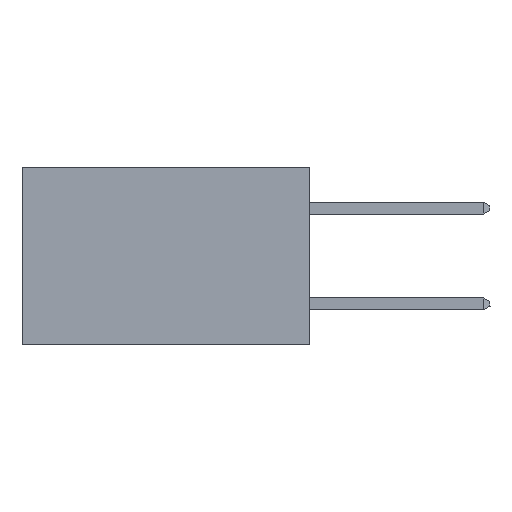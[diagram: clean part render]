
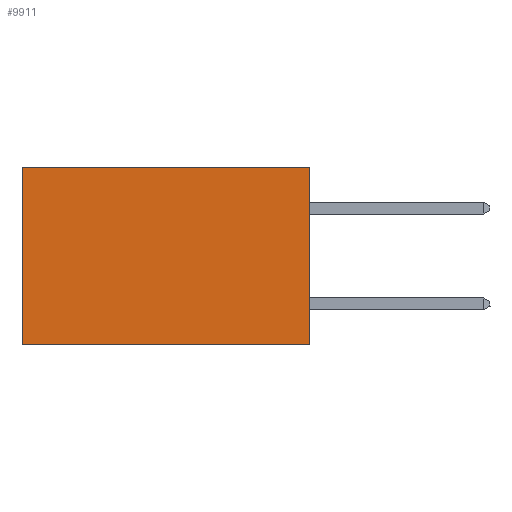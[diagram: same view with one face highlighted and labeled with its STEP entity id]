
A CAD part, left-side view. The second image highlights one B-rep face of the part: STEP entity #9911.
In plain terms, the highlighted planar face has unit normal (-1, 0, 0).
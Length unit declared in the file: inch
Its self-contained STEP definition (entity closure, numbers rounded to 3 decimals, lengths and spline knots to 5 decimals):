
#1926 = VECTOR ( 'NONE', #7332, 39.37008 ) ;
#2102 = EDGE_LOOP ( 'NONE', ( #9820, #22563, #12753, #5628 ) ) ;
#2512 = CARTESIAN_POINT ( 'NONE',  ( 0.2875, 0., 0. ) ) ;
#2703 = VERTEX_POINT ( 'NONE', #6665 ) ;
#3456 = LINE ( 'NONE', #10972, #8650 ) ;
#4264 = EDGE_CURVE ( 'NONE', #2703, #23102, #3456, .T. ) ;
#4873 = CARTESIAN_POINT ( 'NONE',  ( 0.2875, 0.6, -0.37 ) ) ;
#5211 = LINE ( 'NONE', #26821, #21614 ) ;
#5628 = ORIENTED_EDGE ( 'NONE', *, *, #11173, .T. ) ;
#6344 = VECTOR ( 'NONE', #9142, 39.37008 ) ;
#6665 = CARTESIAN_POINT ( 'NONE',  ( 0.2875, 0., -0.37 ) ) ;
#7332 = DIRECTION ( 'NONE',  ( 0., 0., -1. ) ) ;
#8149 = FACE_OUTER_BOUND ( 'NONE', #2102, .T. ) ;
#8650 = VECTOR ( 'NONE', #13106, 39.37008 ) ;
#9142 = DIRECTION ( 'NONE',  ( 0., 1., 0. ) ) ;
#9820 = ORIENTED_EDGE ( 'NONE', *, *, #18787, .T. ) ;
#9911 = ADVANCED_FACE ( 'NONE', ( #8149 ), #19847, .F. ) ;
#10972 = CARTESIAN_POINT ( 'NONE',  ( 0.2875, 0., -0.37 ) ) ;
#11173 = EDGE_CURVE ( 'NONE', #26231, #19776, #12278, .T. ) ;
#12278 = LINE ( 'NONE', #2512, #6344 ) ;
#12753 = ORIENTED_EDGE ( 'NONE', *, *, #16447, .F. ) ;
#13106 = DIRECTION ( 'NONE',  ( 0., 1., 0. ) ) ;
#13458 = DIRECTION ( 'NONE',  ( 0., 0., -1. ) ) ;
#14520 = CARTESIAN_POINT ( 'NONE',  ( 0.2875, 0., 0. ) ) ;
#14707 = AXIS2_PLACEMENT_3D ( 'NONE', #22088, #15084, #21805 ) ;
#15084 = DIRECTION ( 'NONE',  ( 1., 0., 0. ) ) ;
#15489 = LINE ( 'NONE', #20313, #1926 ) ;
#16447 = EDGE_CURVE ( 'NONE', #26231, #2703, #15489, .T. ) ;
#18787 = EDGE_CURVE ( 'NONE', #19776, #23102, #5211, .T. ) ;
#19071 = CARTESIAN_POINT ( 'NONE',  ( 0.2875, 0.6, 0. ) ) ;
#19776 = VERTEX_POINT ( 'NONE', #19071 ) ;
#19847 = PLANE ( 'NONE',  #14707 ) ;
#20313 = CARTESIAN_POINT ( 'NONE',  ( 0.2875, 0., 0. ) ) ;
#21614 = VECTOR ( 'NONE', #13458, 39.37008 ) ;
#21805 = DIRECTION ( 'NONE',  ( 0., 0., -1. ) ) ;
#22088 = CARTESIAN_POINT ( 'NONE',  ( 0.2875, 0., 0. ) ) ;
#22563 = ORIENTED_EDGE ( 'NONE', *, *, #4264, .F. ) ;
#23102 = VERTEX_POINT ( 'NONE', #4873 ) ;
#26231 = VERTEX_POINT ( 'NONE', #14520 ) ;
#26821 = CARTESIAN_POINT ( 'NONE',  ( 0.2875, 0.6, 0. ) ) ;
